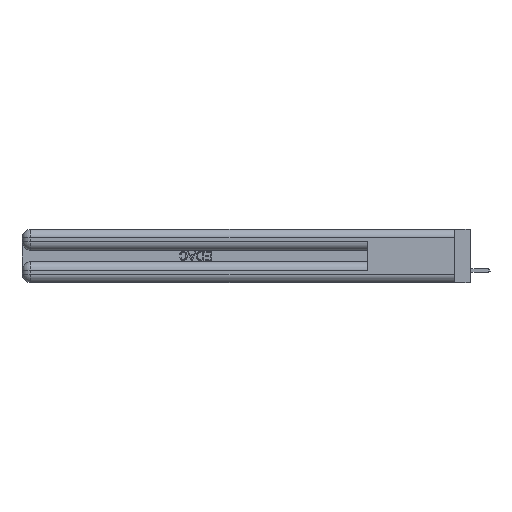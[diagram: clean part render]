
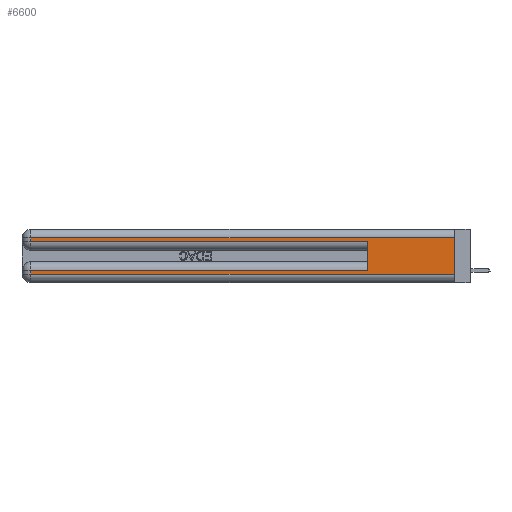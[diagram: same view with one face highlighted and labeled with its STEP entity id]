
A CAD part, left-side view. The second image highlights one B-rep face of the part: STEP entity #6600.
In plain terms, the highlighted planar face has unit normal (-1, 0, 0).
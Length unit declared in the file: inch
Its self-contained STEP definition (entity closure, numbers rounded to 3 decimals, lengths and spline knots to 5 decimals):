
#615 = DIRECTION ( 'NONE',  ( 0., 0., -1. ) ) ;
#959 = EDGE_CURVE ( 'NONE', #12227, #42654, #43365, .T. ) ;
#2020 = ORIENTED_EDGE ( 'NONE', *, *, #5822, .T. ) ;
#2649 = EDGE_CURVE ( 'NONE', #7997, #41956, #11060, .T. ) ;
#5822 = EDGE_CURVE ( 'NONE', #9784, #7997, #6934, .T. ) ;
#6600 = ADVANCED_FACE ( 'NONE', ( #33405 ), #9936, .F. ) ;
#6934 = LINE ( 'NONE', #27146, #34037 ) ;
#7485 = CARTESIAN_POINT ( 'NONE',  ( 0., 0., 0.37 ) ) ;
#7669 = CARTESIAN_POINT ( 'NONE',  ( 0., 2.94, 0.085 ) ) ;
#7997 = VERTEX_POINT ( 'NONE', #39736 ) ;
#9318 = CARTESIAN_POINT ( 'NONE',  ( 0., 0., 0.31 ) ) ;
#9634 = DIRECTION ( 'NONE',  ( 1., 0., 0. ) ) ;
#9784 = VERTEX_POINT ( 'NONE', #7669 ) ;
#9936 = PLANE ( 'NONE',  #39066 ) ;
#11060 = LINE ( 'NONE', #32949, #22465 ) ;
#12227 = VERTEX_POINT ( 'NONE', #28179 ) ;
#12527 = LINE ( 'NONE', #9318, #20717 ) ;
#13041 = EDGE_CURVE ( 'NONE', #41371, #19311, #17126, .T. ) ;
#13049 = CARTESIAN_POINT ( 'NONE',  ( 0., 0., 0.085 ) ) ;
#13565 = CARTESIAN_POINT ( 'NONE',  ( 0., 0., 0.06 ) ) ;
#15912 = ORIENTED_EDGE ( 'NONE', *, *, #13041, .T. ) ;
#16083 = VERTEX_POINT ( 'NONE', #18863 ) ;
#16651 = EDGE_CURVE ( 'NONE', #12227, #9784, #35504, .T. ) ;
#17126 = LINE ( 'NONE', #24636, #44279 ) ;
#17399 = EDGE_CURVE ( 'NONE', #16083, #41956, #21918, .T. ) ;
#17965 = CARTESIAN_POINT ( 'NONE',  ( 0., 2.94, 0.285 ) ) ;
#18253 = DIRECTION ( 'NONE',  ( 0., -1., 0. ) ) ;
#18863 = CARTESIAN_POINT ( 'NONE',  ( 0., 0., 0.31 ) ) ;
#19050 = DIRECTION ( 'NONE',  ( 0., 0., 1. ) ) ;
#19311 = VERTEX_POINT ( 'NONE', #17965 ) ;
#19724 = LINE ( 'NONE', #24830, #30045 ) ;
#19841 = DIRECTION ( 'NONE',  ( 0., 0., -1. ) ) ;
#20717 = VECTOR ( 'NONE', #22506, 39.37008 ) ;
#21157 = DIRECTION ( 'NONE',  ( 0., 0., -1. ) ) ;
#21918 = LINE ( 'NONE', #7485, #39250 ) ;
#22465 = VECTOR ( 'NONE', #43450, 39.37008 ) ;
#22506 = DIRECTION ( 'NONE',  ( 0., 1., 0. ) ) ;
#24636 = CARTESIAN_POINT ( 'NONE',  ( 0., 2.94, 0.37 ) ) ;
#24830 = CARTESIAN_POINT ( 'NONE',  ( 0., 0., 0.285 ) ) ;
#26924 = ORIENTED_EDGE ( 'NONE', *, *, #30076, .T. ) ;
#27146 = CARTESIAN_POINT ( 'NONE',  ( 0., 2.94, 0.37 ) ) ;
#28179 = CARTESIAN_POINT ( 'NONE',  ( 0., 0.6, 0.085 ) ) ;
#30045 = VECTOR ( 'NONE', #18253, 39.37008 ) ;
#30076 = EDGE_CURVE ( 'NONE', #19311, #42654, #19724, .T. ) ;
#30190 = DIRECTION ( 'NONE',  ( 0., 1., 0. ) ) ;
#30224 = CARTESIAN_POINT ( 'NONE',  ( 0., 0., 0.37 ) ) ;
#31644 = ORIENTED_EDGE ( 'NONE', *, *, #35419, .T. ) ;
#31932 = VECTOR ( 'NONE', #19050, 39.37008 ) ;
#32949 = CARTESIAN_POINT ( 'NONE',  ( 0., 0., 0.06 ) ) ;
#33328 = VECTOR ( 'NONE', #30190, 39.37008 ) ;
#33405 = FACE_OUTER_BOUND ( 'NONE', #35146, .T. ) ;
#34037 = VECTOR ( 'NONE', #19841, 39.37008 ) ;
#35146 = EDGE_LOOP ( 'NONE', ( #40649, #31644, #15912, #26924, #42861, #43844, #2020, #42578 ) ) ;
#35419 = EDGE_CURVE ( 'NONE', #16083, #41371, #12527, .T. ) ;
#35504 = LINE ( 'NONE', #13049, #33328 ) ;
#39066 = AXIS2_PLACEMENT_3D ( 'NONE', #30224, #9634, #41034 ) ;
#39250 = VECTOR ( 'NONE', #615, 39.37008 ) ;
#39736 = CARTESIAN_POINT ( 'NONE',  ( 0., 2.94, 0.06 ) ) ;
#39863 = CARTESIAN_POINT ( 'NONE',  ( 0., 0.6, 0.145 ) ) ;
#40649 = ORIENTED_EDGE ( 'NONE', *, *, #17399, .F. ) ;
#41034 = DIRECTION ( 'NONE',  ( 0., 0., -1. ) ) ;
#41102 = CARTESIAN_POINT ( 'NONE',  ( 0., 2.94, 0.31 ) ) ;
#41298 = CARTESIAN_POINT ( 'NONE',  ( 0., 0.6, 0.285 ) ) ;
#41371 = VERTEX_POINT ( 'NONE', #41102 ) ;
#41956 = VERTEX_POINT ( 'NONE', #13565 ) ;
#42578 = ORIENTED_EDGE ( 'NONE', *, *, #2649, .T. ) ;
#42654 = VERTEX_POINT ( 'NONE', #41298 ) ;
#42861 = ORIENTED_EDGE ( 'NONE', *, *, #959, .F. ) ;
#43365 = LINE ( 'NONE', #39863, #31932 ) ;
#43450 = DIRECTION ( 'NONE',  ( 0., -1., 0. ) ) ;
#43844 = ORIENTED_EDGE ( 'NONE', *, *, #16651, .T. ) ;
#44279 = VECTOR ( 'NONE', #21157, 39.37008 ) ;
